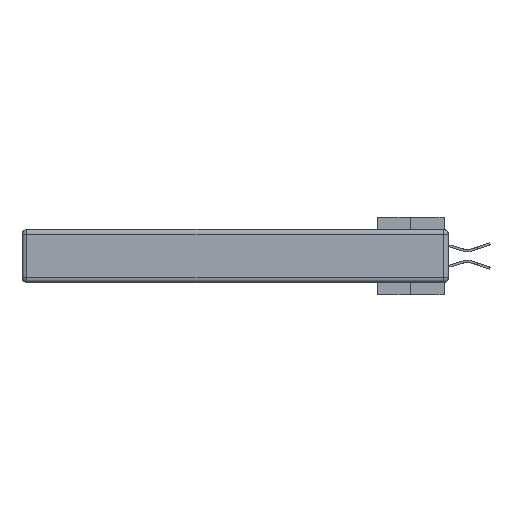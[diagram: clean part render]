
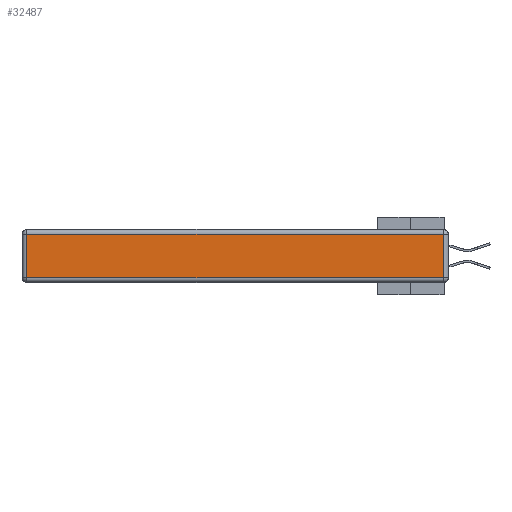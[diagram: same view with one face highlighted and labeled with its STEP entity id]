
A CAD part, left-side view. The second image highlights one B-rep face of the part: STEP entity #32487.
In plain terms, the highlighted planar face has unit normal (-1, 0, 0).
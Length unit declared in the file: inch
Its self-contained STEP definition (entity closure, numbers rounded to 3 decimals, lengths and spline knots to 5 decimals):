
#66 = LINE ( 'NONE', #9893, #10979 ) ;
#877 = PLANE ( 'NONE',  #8743 ) ;
#1471 = LINE ( 'NONE', #37220, #22415 ) ;
#1472 = DIRECTION ( 'NONE',  ( 0., 1., 0. ) ) ;
#5958 = VERTEX_POINT ( 'NONE', #37229 ) ;
#7207 = VECTOR ( 'NONE', #1472, 39.37008 ) ;
#8735 = DIRECTION ( 'NONE',  ( 0., 0., -1. ) ) ;
#8743 = AXIS2_PLACEMENT_3D ( 'NONE', #10599, #39090, #16982 ) ;
#9893 = CARTESIAN_POINT ( 'NONE',  ( 0., 0.03, -0.343 ) ) ;
#10599 = CARTESIAN_POINT ( 'NONE',  ( 0., 0., -0.343 ) ) ;
#10979 = VECTOR ( 'NONE', #12960, 39.37008 ) ;
#12765 = LINE ( 'NONE', #41090, #16689 ) ;
#12960 = DIRECTION ( 'NONE',  ( 0., 0., 1. ) ) ;
#15636 = EDGE_CURVE ( 'NONE', #5958, #21129, #12765, .T. ) ;
#15726 = ORIENTED_EDGE ( 'NONE', *, *, #15636, .T. ) ;
#16689 = VECTOR ( 'NONE', #22202, 39.37008 ) ;
#16982 = DIRECTION ( 'NONE',  ( 0., 0., 1. ) ) ;
#19159 = LINE ( 'NONE', #36640, #7207 ) ;
#20890 = EDGE_LOOP ( 'NONE', ( #15726, #26554, #26983, #38222 ) ) ;
#21129 = VERTEX_POINT ( 'NONE', #30807 ) ;
#21462 = VERTEX_POINT ( 'NONE', #23392 ) ;
#21707 = VERTEX_POINT ( 'NONE', #31745 ) ;
#22202 = DIRECTION ( 'NONE',  ( 0., -1., 0. ) ) ;
#22415 = VECTOR ( 'NONE', #8735, 39.37008 ) ;
#23392 = CARTESIAN_POINT ( 'NONE',  ( 0., 0.03, -0.03 ) ) ;
#23446 = EDGE_CURVE ( 'NONE', #21129, #21462, #66, .T. ) ;
#26554 = ORIENTED_EDGE ( 'NONE', *, *, #23446, .T. ) ;
#26983 = ORIENTED_EDGE ( 'NONE', *, *, #29328, .T. ) ;
#29328 = EDGE_CURVE ( 'NONE', #21462, #21707, #19159, .T. ) ;
#30807 = CARTESIAN_POINT ( 'NONE',  ( 0., 0.03, -0.313 ) ) ;
#31745 = CARTESIAN_POINT ( 'NONE',  ( 0., 2.72, -0.03 ) ) ;
#32487 = ADVANCED_FACE ( 'NONE', ( #32750 ), #877, .T. ) ;
#32750 = FACE_OUTER_BOUND ( 'NONE', #20890, .T. ) ;
#36640 = CARTESIAN_POINT ( 'NONE',  ( 0., 2.75, -0.03 ) ) ;
#37220 = CARTESIAN_POINT ( 'NONE',  ( 0., 2.72, -0.343 ) ) ;
#37229 = CARTESIAN_POINT ( 'NONE',  ( 0., 2.72, -0.313 ) ) ;
#38222 = ORIENTED_EDGE ( 'NONE', *, *, #40654, .T. ) ;
#39090 = DIRECTION ( 'NONE',  ( -1., 0., 0. ) ) ;
#40654 = EDGE_CURVE ( 'NONE', #21707, #5958, #1471, .T. ) ;
#41090 = CARTESIAN_POINT ( 'NONE',  ( 0., 0., -0.313 ) ) ;
